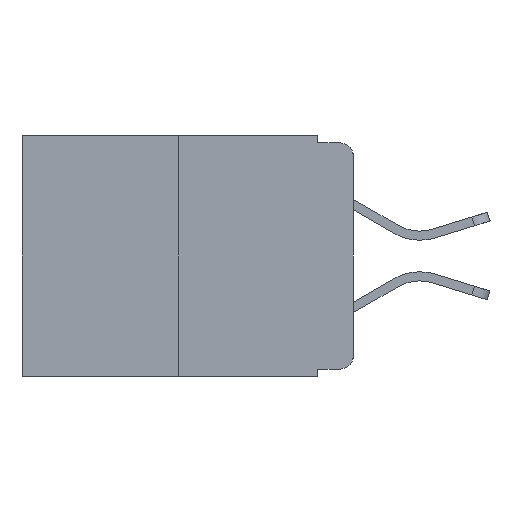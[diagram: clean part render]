
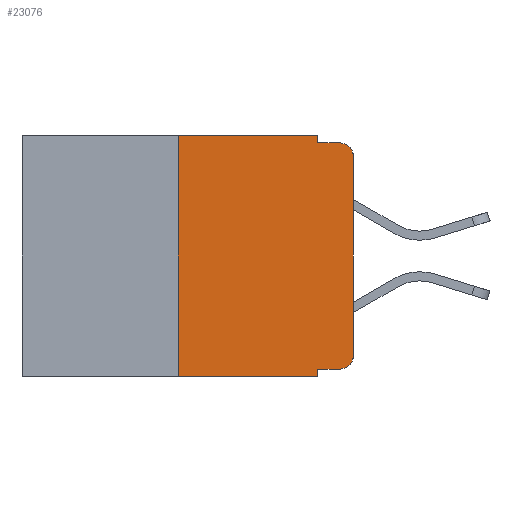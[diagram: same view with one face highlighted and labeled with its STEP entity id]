
A CAD part, left-side view. The second image highlights one B-rep face of the part: STEP entity #23076.
In plain terms, the highlighted planar face has unit normal (-1, 0, 0).
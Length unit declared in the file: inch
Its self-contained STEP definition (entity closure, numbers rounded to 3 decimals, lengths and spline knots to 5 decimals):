
#72 = AXIS2_PLACEMENT_3D ( 'NONE', #16440, #5813, #18223 ) ;
#102 = VERTEX_POINT ( 'NONE', #20605 ) ;
#246 = DIRECTION ( 'NONE',  ( 0., 0., 1. ) ) ;
#298 = VECTOR ( 'NONE', #1400, 39.37008 ) ;
#573 = ORIENTED_EDGE ( 'NONE', *, *, #13278, .T. ) ;
#776 = DIRECTION ( 'NONE',  ( 0., 0., -1. ) ) ;
#1173 = CARTESIAN_POINT ( 'NONE',  ( 0., 0.02, -0.01 ) ) ;
#1400 = DIRECTION ( 'NONE',  ( 0., -1., 0. ) ) ;
#1667 = CARTESIAN_POINT ( 'NONE',  ( 0., 0.25, 0. ) ) ;
#1853 = EDGE_CURVE ( 'NONE', #21943, #14185, #3839, .T. ) ;
#1890 = VECTOR ( 'NONE', #18619, 39.37008 ) ;
#2349 = CARTESIAN_POINT ( 'NONE',  ( 0., 0.473, 0. ) ) ;
#2619 = CARTESIAN_POINT ( 'NONE',  ( 0., 0.051, -0.01 ) ) ;
#3369 = CARTESIAN_POINT ( 'NONE',  ( 0., 0.25, 0. ) ) ;
#3514 = ORIENTED_EDGE ( 'NONE', *, *, #5155, .F. ) ;
#3839 = LINE ( 'NONE', #3369, #18637 ) ;
#4520 = CARTESIAN_POINT ( 'NONE',  ( 0., 0.02, -0.333 ) ) ;
#4685 = EDGE_CURVE ( 'NONE', #15098, #9277, #6598, .T. ) ;
#4803 = AXIS2_PLACEMENT_3D ( 'NONE', #22268, #11725, #776 ) ;
#5155 = EDGE_CURVE ( 'NONE', #22824, #9877, #14912, .T. ) ;
#5483 = AXIS2_PLACEMENT_3D ( 'NONE', #21031, #10460, #22781 ) ;
#5580 = ORIENTED_EDGE ( 'NONE', *, *, #4685, .T. ) ;
#5813 = DIRECTION ( 'NONE',  ( 1., 0., 0. ) ) ;
#6017 = VECTOR ( 'NONE', #14290, 39.37008 ) ;
#6198 = CARTESIAN_POINT ( 'NONE',  ( 0., 0.051, 0. ) ) ;
#6598 = LINE ( 'NONE', #16129, #6017 ) ;
#6747 = ORIENTED_EDGE ( 'NONE', *, *, #9971, .T. ) ;
#6817 = LINE ( 'NONE', #6198, #1890 ) ;
#6820 = EDGE_CURVE ( 'NONE', #102, #10575, #6817, .T. ) ;
#7050 = ORIENTED_EDGE ( 'NONE', *, *, #8449, .F. ) ;
#7101 = ORIENTED_EDGE ( 'NONE', *, *, #1853, .F. ) ;
#7211 = ORIENTED_EDGE ( 'NONE', *, *, #6820, .F. ) ;
#7351 = LINE ( 'NONE', #2349, #16186 ) ;
#7652 = ORIENTED_EDGE ( 'NONE', *, *, #16309, .T. ) ;
#8361 = ORIENTED_EDGE ( 'NONE', *, *, #14757, .T. ) ;
#8449 = EDGE_CURVE ( 'NONE', #14185, #102, #7351, .T. ) ;
#8578 = VECTOR ( 'NONE', #15559, 39.37008 ) ;
#8942 = CARTESIAN_POINT ( 'NONE',  ( 0., 0.051, 0. ) ) ;
#9277 = VERTEX_POINT ( 'NONE', #12025 ) ;
#9718 = CARTESIAN_POINT ( 'NONE',  ( 0., 0.051, -0.343 ) ) ;
#9877 = VERTEX_POINT ( 'NONE', #9718 ) ;
#9971 = EDGE_CURVE ( 'NONE', #22824, #15856, #21651, .T. ) ;
#10326 = CARTESIAN_POINT ( 'NONE',  ( 0., 0.051, -0.01 ) ) ;
#10460 = DIRECTION ( 'NONE',  ( -1., 0., 0. ) ) ;
#10575 = VERTEX_POINT ( 'NONE', #2619 ) ;
#11136 = PLANE ( 'NONE',  #72 ) ;
#11725 = DIRECTION ( 'NONE',  ( -1., 0., 0. ) ) ;
#11728 = CARTESIAN_POINT ( 'NONE',  ( 0., 0.051, -0.333 ) ) ;
#12025 = CARTESIAN_POINT ( 'NONE',  ( 0., 0., -0.03 ) ) ;
#13125 = ORIENTED_EDGE ( 'NONE', *, *, #17508, .F. ) ;
#13278 = EDGE_CURVE ( 'NONE', #15856, #15098, #13466, .T. ) ;
#13466 = CIRCLE ( 'NONE', #4803, 0.02 ) ;
#13494 = DIRECTION ( 'NONE',  ( 0., -1., 0. ) ) ;
#14122 = DIRECTION ( 'NONE',  ( 0., 0., -1. ) ) ;
#14185 = VERTEX_POINT ( 'NONE', #1667 ) ;
#14290 = DIRECTION ( 'NONE',  ( 0., 0., 1. ) ) ;
#14757 = EDGE_CURVE ( 'NONE', #21943, #9877, #19484, .T. ) ;
#14820 = FACE_OUTER_BOUND ( 'NONE', #19106, .T. ) ;
#14877 = CARTESIAN_POINT ( 'NONE',  ( 0., 0., -0.313 ) ) ;
#14912 = LINE ( 'NONE', #8942, #19611 ) ;
#15098 = VERTEX_POINT ( 'NONE', #14877 ) ;
#15271 = CIRCLE ( 'NONE', #5483, 0.02 ) ;
#15559 = DIRECTION ( 'NONE',  ( 0., -1., 0. ) ) ;
#15856 = VERTEX_POINT ( 'NONE', #4520 ) ;
#16129 = CARTESIAN_POINT ( 'NONE',  ( 0., 0., 0. ) ) ;
#16186 = VECTOR ( 'NONE', #18543, 39.37008 ) ;
#16309 = EDGE_CURVE ( 'NONE', #9277, #22782, #15271, .T. ) ;
#16392 = VECTOR ( 'NONE', #13494, 39.37008 ) ;
#16415 = CARTESIAN_POINT ( 'NONE',  ( 0., 0.25, -0.343 ) ) ;
#16440 = CARTESIAN_POINT ( 'NONE',  ( 0., 0.473, 0. ) ) ;
#17508 = EDGE_CURVE ( 'NONE', #10575, #22782, #22636, .T. ) ;
#18223 = DIRECTION ( 'NONE',  ( 0., 0., -1. ) ) ;
#18543 = DIRECTION ( 'NONE',  ( 0., -1., 0. ) ) ;
#18619 = DIRECTION ( 'NONE',  ( 0., 0., -1. ) ) ;
#18637 = VECTOR ( 'NONE', #246, 39.37008 ) ;
#19106 = EDGE_LOOP ( 'NONE', ( #5580, #7652, #13125, #7211, #7050, #7101, #8361, #3514, #6747, #573 ) ) ;
#19484 = LINE ( 'NONE', #22746, #298 ) ;
#19611 = VECTOR ( 'NONE', #14122, 39.37008 ) ;
#20605 = CARTESIAN_POINT ( 'NONE',  ( 0., 0.051, 0. ) ) ;
#21031 = CARTESIAN_POINT ( 'NONE',  ( 0., 0.02, -0.03 ) ) ;
#21651 = LINE ( 'NONE', #11728, #16392 ) ;
#21943 = VERTEX_POINT ( 'NONE', #16415 ) ;
#22268 = CARTESIAN_POINT ( 'NONE',  ( 0., 0.02, -0.313 ) ) ;
#22636 = LINE ( 'NONE', #10326, #8578 ) ;
#22746 = CARTESIAN_POINT ( 'NONE',  ( 0., 0.473, -0.343 ) ) ;
#22779 = CARTESIAN_POINT ( 'NONE',  ( 0., 0.051, -0.333 ) ) ;
#22781 = DIRECTION ( 'NONE',  ( 0., 0., -1. ) ) ;
#22782 = VERTEX_POINT ( 'NONE', #1173 ) ;
#22824 = VERTEX_POINT ( 'NONE', #22779 ) ;
#23076 = ADVANCED_FACE ( 'NONE', ( #14820 ), #11136, .F. ) ;
